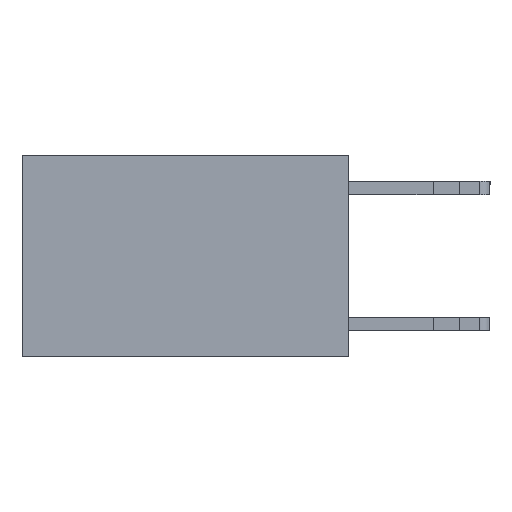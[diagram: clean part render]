
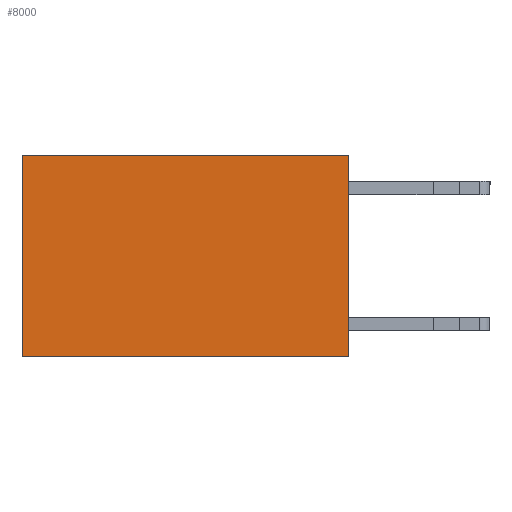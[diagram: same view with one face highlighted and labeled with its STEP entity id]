
A CAD part, left-side view. The second image highlights one B-rep face of the part: STEP entity #8000.
In plain terms, the highlighted planar face has unit normal (-1, 0, 0).
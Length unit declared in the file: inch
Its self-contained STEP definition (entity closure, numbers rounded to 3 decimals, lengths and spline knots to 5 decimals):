
#223 = VERTEX_POINT ( 'NONE', #10031 ) ;
#244 = EDGE_CURVE ( 'NONE', #5230, #18081, #8468, .T. ) ;
#918 = DIRECTION ( 'NONE',  ( 0., 0., -1. ) ) ;
#1130 = DIRECTION ( 'NONE',  ( 0., 0., -1. ) ) ;
#3140 = VECTOR ( 'NONE', #11515, 39.37008 ) ;
#3495 = LINE ( 'NONE', #11206, #10764 ) ;
#3962 = LINE ( 'NONE', #9909, #6772 ) ;
#4011 = VECTOR ( 'NONE', #918, 39.37008 ) ;
#4938 = EDGE_LOOP ( 'NONE', ( #10471, #19033, #15023, #14971 ) ) ;
#4994 = LINE ( 'NONE', #11048, #4011 ) ;
#5230 = VERTEX_POINT ( 'NONE', #11007 ) ;
#6772 = VECTOR ( 'NONE', #1130, 39.37008 ) ;
#7416 = CARTESIAN_POINT ( 'NONE',  ( 0.2625, 0., 0. ) ) ;
#7503 = DIRECTION ( 'NONE',  ( 1., 0., 0. ) ) ;
#8000 = ADVANCED_FACE ( 'NONE', ( #19292 ), #17484, .F. ) ;
#8468 = LINE ( 'NONE', #12970, #3140 ) ;
#8786 = EDGE_CURVE ( 'NONE', #18658, #223, #3495, .T. ) ;
#8858 = AXIS2_PLACEMENT_3D ( 'NONE', #7416, #7503, #10347 ) ;
#9909 = CARTESIAN_POINT ( 'NONE',  ( 0.2625, 0.6, 0. ) ) ;
#10031 = CARTESIAN_POINT ( 'NONE',  ( 0.2625, 0.6, 0. ) ) ;
#10347 = DIRECTION ( 'NONE',  ( 0., 0., -1. ) ) ;
#10471 = ORIENTED_EDGE ( 'NONE', *, *, #16254, .T. ) ;
#10764 = VECTOR ( 'NONE', #15698, 39.37008 ) ;
#11007 = CARTESIAN_POINT ( 'NONE',  ( 0.2625, 0., -0.37 ) ) ;
#11048 = CARTESIAN_POINT ( 'NONE',  ( 0.2625, 0., 0. ) ) ;
#11206 = CARTESIAN_POINT ( 'NONE',  ( 0.2625, 0., 0. ) ) ;
#11515 = DIRECTION ( 'NONE',  ( 0., 1., 0. ) ) ;
#12970 = CARTESIAN_POINT ( 'NONE',  ( 0.2625, 0., -0.37 ) ) ;
#14971 = ORIENTED_EDGE ( 'NONE', *, *, #8786, .T. ) ;
#15023 = ORIENTED_EDGE ( 'NONE', *, *, #15258, .F. ) ;
#15258 = EDGE_CURVE ( 'NONE', #18658, #5230, #4994, .T. ) ;
#15698 = DIRECTION ( 'NONE',  ( 0., 1., 0. ) ) ;
#16071 = CARTESIAN_POINT ( 'NONE',  ( 0.2625, 0.6, -0.37 ) ) ;
#16254 = EDGE_CURVE ( 'NONE', #223, #18081, #3962, .T. ) ;
#17484 = PLANE ( 'NONE',  #8858 ) ;
#17877 = CARTESIAN_POINT ( 'NONE',  ( 0.2625, 0., 0. ) ) ;
#18081 = VERTEX_POINT ( 'NONE', #16071 ) ;
#18658 = VERTEX_POINT ( 'NONE', #17877 ) ;
#19033 = ORIENTED_EDGE ( 'NONE', *, *, #244, .F. ) ;
#19292 = FACE_OUTER_BOUND ( 'NONE', #4938, .T. ) ;
